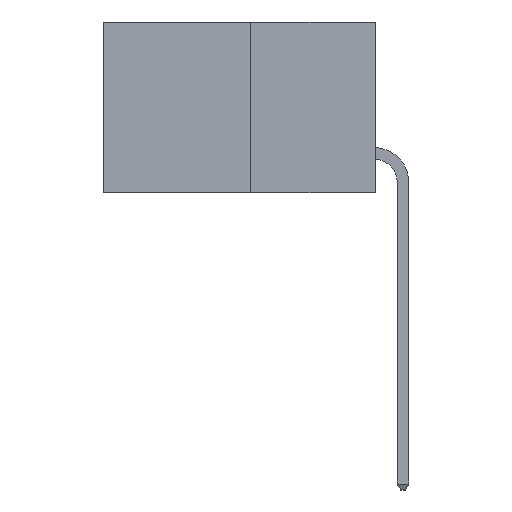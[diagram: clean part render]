
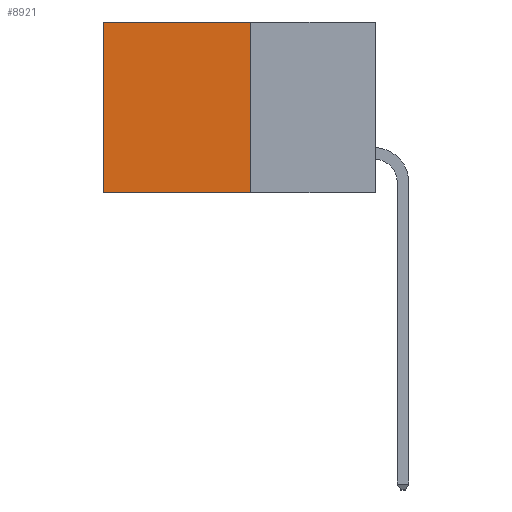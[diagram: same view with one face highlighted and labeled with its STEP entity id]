
A CAD part, left-side view. The second image highlights one B-rep face of the part: STEP entity #8921.
In plain terms, the highlighted planar face has unit normal (-1, 0, 0).
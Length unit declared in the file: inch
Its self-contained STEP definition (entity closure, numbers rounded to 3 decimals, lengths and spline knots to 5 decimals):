
#342 = VERTEX_POINT ( 'NONE', #2191 ) ;
#813 = LINE ( 'NONE', #4331, #6780 ) ;
#1196 = LINE ( 'NONE', #7135, #8994 ) ;
#1292 = DIRECTION ( 'NONE',  ( 1., 0., 0. ) ) ;
#1346 = VERTEX_POINT ( 'NONE', #2245 ) ;
#1822 = EDGE_CURVE ( 'NONE', #9070, #342, #6127, .T. ) ;
#2191 = CARTESIAN_POINT ( 'NONE',  ( 0.277, 0.27, -0.37 ) ) ;
#2245 = CARTESIAN_POINT ( 'NONE',  ( 0.277, 0.59, -0.37 ) ) ;
#2429 = DIRECTION ( 'NONE',  ( 0., 1., 0. ) ) ;
#3937 = ORIENTED_EDGE ( 'NONE', *, *, #4832, .T. ) ;
#3959 = CARTESIAN_POINT ( 'NONE',  ( 0.277, 0.27, 0. ) ) ;
#4331 = CARTESIAN_POINT ( 'NONE',  ( 0.277, 0.27, -0.37 ) ) ;
#4366 = DIRECTION ( 'NONE',  ( 0., 1., 0. ) ) ;
#4472 = PLANE ( 'NONE',  #8090 ) ;
#4832 = EDGE_CURVE ( 'NONE', #8171, #1346, #1196, .T. ) ;
#5210 = CARTESIAN_POINT ( 'NONE',  ( 0.277, 0.27, -0.37 ) ) ;
#5622 = CARTESIAN_POINT ( 'NONE',  ( 0.277, 0.27, -0.37 ) ) ;
#5657 = EDGE_LOOP ( 'NONE', ( #3937, #9564, #7651, #6507 ) ) ;
#5992 = DIRECTION ( 'NONE',  ( 0., 0., -1. ) ) ;
#6127 = LINE ( 'NONE', #5622, #6357 ) ;
#6154 = CARTESIAN_POINT ( 'NONE',  ( 0.277, 0.27, 0. ) ) ;
#6357 = VECTOR ( 'NONE', #5992, 39.37008 ) ;
#6507 = ORIENTED_EDGE ( 'NONE', *, *, #8494, .T. ) ;
#6683 = DIRECTION ( 'NONE',  ( 0., 0., -1. ) ) ;
#6687 = EDGE_CURVE ( 'NONE', #342, #1346, #813, .T. ) ;
#6780 = VECTOR ( 'NONE', #4366, 39.37008 ) ;
#7135 = CARTESIAN_POINT ( 'NONE',  ( 0.277, 0.59, -0.37 ) ) ;
#7651 = ORIENTED_EDGE ( 'NONE', *, *, #1822, .F. ) ;
#7898 = VECTOR ( 'NONE', #2429, 39.37008 ) ;
#8088 = FACE_OUTER_BOUND ( 'NONE', #5657, .T. ) ;
#8090 = AXIS2_PLACEMENT_3D ( 'NONE', #5210, #1292, #6683 ) ;
#8171 = VERTEX_POINT ( 'NONE', #8727 ) ;
#8494 = EDGE_CURVE ( 'NONE', #9070, #8171, #9778, .T. ) ;
#8727 = CARTESIAN_POINT ( 'NONE',  ( 0.277, 0.59, 0. ) ) ;
#8921 = ADVANCED_FACE ( 'NONE', ( #8088 ), #4472, .F. ) ;
#8994 = VECTOR ( 'NONE', #9740, 39.37008 ) ;
#9070 = VERTEX_POINT ( 'NONE', #6154 ) ;
#9564 = ORIENTED_EDGE ( 'NONE', *, *, #6687, .F. ) ;
#9740 = DIRECTION ( 'NONE',  ( 0., 0., -1. ) ) ;
#9778 = LINE ( 'NONE', #3959, #7898 ) ;
